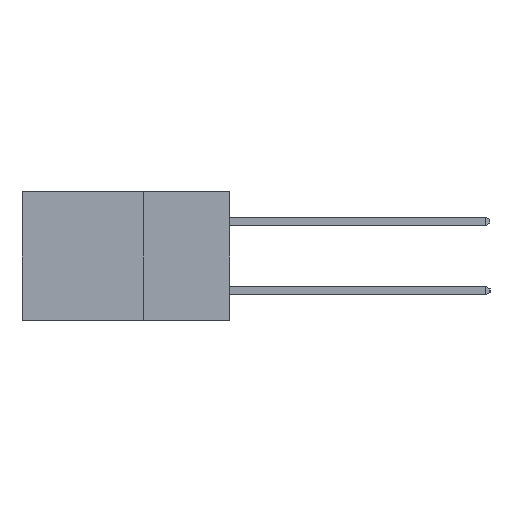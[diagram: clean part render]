
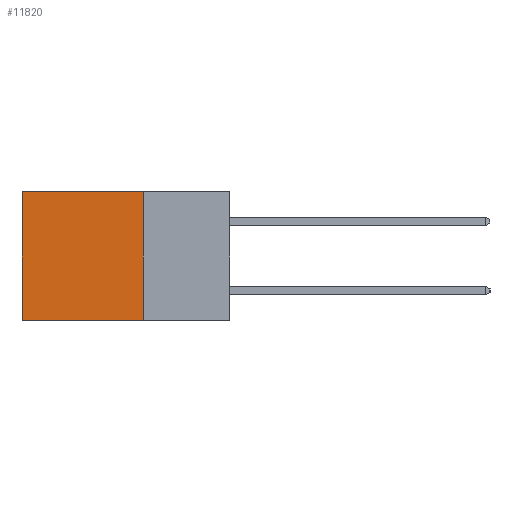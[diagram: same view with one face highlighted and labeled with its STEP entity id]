
A CAD part, left-side view. The second image highlights one B-rep face of the part: STEP entity #11820.
In plain terms, the highlighted planar face has unit normal (-1, 0, 0).
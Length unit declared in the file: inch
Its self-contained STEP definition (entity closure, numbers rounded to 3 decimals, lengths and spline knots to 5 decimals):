
#40 = AXIS2_PLACEMENT_3D ( 'NONE', #3368, #9875, #4281 ) ;
#120 = EDGE_CURVE ( 'NONE', #1142, #9205, #4972, .T. ) ;
#800 = CARTESIAN_POINT ( 'NONE',  ( 0.2615, 0.25, -0.37 ) ) ;
#1129 = EDGE_LOOP ( 'NONE', ( #5772, #7928, #11051, #6528 ) ) ;
#1142 = VERTEX_POINT ( 'NONE', #800 ) ;
#1168 = CARTESIAN_POINT ( 'NONE',  ( 0.2615, 0.6, -0.37 ) ) ;
#1442 = DIRECTION ( 'NONE',  ( 0., 1., 0. ) ) ;
#1496 = LINE ( 'NONE', #3990, #11161 ) ;
#2494 = VERTEX_POINT ( 'NONE', #2812 ) ;
#2496 = CARTESIAN_POINT ( 'NONE',  ( 0.2615, 0.6, -0.37 ) ) ;
#2812 = CARTESIAN_POINT ( 'NONE',  ( 0.2615, 0.25, 0. ) ) ;
#3368 = CARTESIAN_POINT ( 'NONE',  ( 0.2615, 0.25, -0.37 ) ) ;
#3715 = VECTOR ( 'NONE', #9950, 39.37008 ) ;
#3990 = CARTESIAN_POINT ( 'NONE',  ( 0.2615, 0.25, -0.37 ) ) ;
#4159 = VERTEX_POINT ( 'NONE', #8009 ) ;
#4281 = DIRECTION ( 'NONE',  ( 0., 0., -1. ) ) ;
#4972 = LINE ( 'NONE', #7563, #9636 ) ;
#5447 = CARTESIAN_POINT ( 'NONE',  ( 0.2615, 0.25, 0. ) ) ;
#5772 = ORIENTED_EDGE ( 'NONE', *, *, #9467, .T. ) ;
#6138 = PLANE ( 'NONE',  #40 ) ;
#6528 = ORIENTED_EDGE ( 'NONE', *, *, #11256, .T. ) ;
#7563 = CARTESIAN_POINT ( 'NONE',  ( 0.2615, 0.25, -0.37 ) ) ;
#7597 = VECTOR ( 'NONE', #11912, 39.37008 ) ;
#7928 = ORIENTED_EDGE ( 'NONE', *, *, #120, .F. ) ;
#7957 = EDGE_CURVE ( 'NONE', #2494, #1142, #1496, .T. ) ;
#8009 = CARTESIAN_POINT ( 'NONE',  ( 0.2615, 0.6, 0. ) ) ;
#9205 = VERTEX_POINT ( 'NONE', #1168 ) ;
#9467 = EDGE_CURVE ( 'NONE', #4159, #9205, #11398, .T. ) ;
#9565 = DIRECTION ( 'NONE',  ( 0., 0., -1. ) ) ;
#9636 = VECTOR ( 'NONE', #1442, 39.37008 ) ;
#9875 = DIRECTION ( 'NONE',  ( 1., 0., 0. ) ) ;
#9950 = DIRECTION ( 'NONE',  ( 0., 0., -1. ) ) ;
#11051 = ORIENTED_EDGE ( 'NONE', *, *, #7957, .F. ) ;
#11161 = VECTOR ( 'NONE', #9565, 39.37008 ) ;
#11256 = EDGE_CURVE ( 'NONE', #2494, #4159, #12200, .T. ) ;
#11398 = LINE ( 'NONE', #2496, #3715 ) ;
#11623 = FACE_OUTER_BOUND ( 'NONE', #1129, .T. ) ;
#11820 = ADVANCED_FACE ( 'NONE', ( #11623 ), #6138, .F. ) ;
#11912 = DIRECTION ( 'NONE',  ( 0., 1., 0. ) ) ;
#12200 = LINE ( 'NONE', #5447, #7597 ) ;
